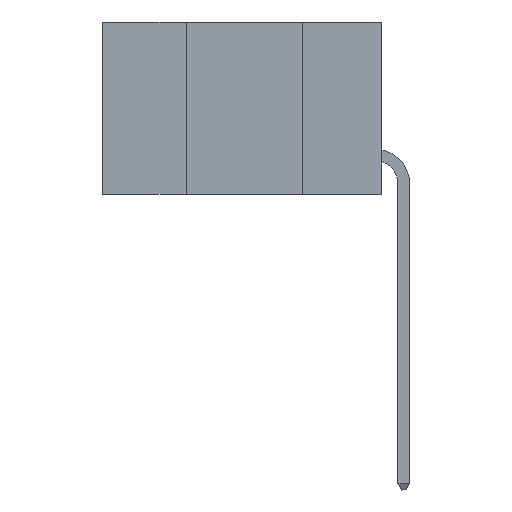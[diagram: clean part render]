
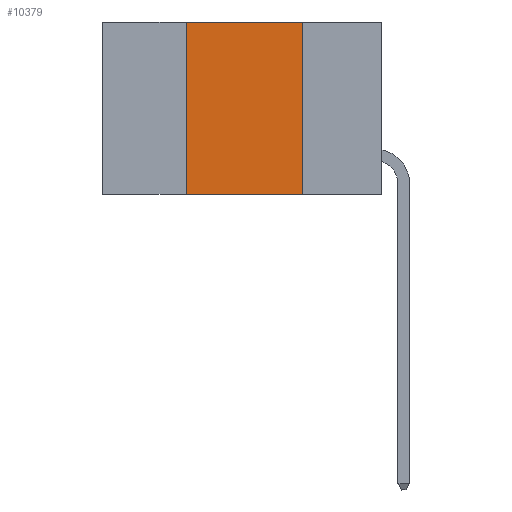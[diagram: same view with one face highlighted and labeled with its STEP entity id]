
A CAD part, left-side view. The second image highlights one B-rep face of the part: STEP entity #10379.
In plain terms, the highlighted planar face has unit normal (-1, 0, 0).
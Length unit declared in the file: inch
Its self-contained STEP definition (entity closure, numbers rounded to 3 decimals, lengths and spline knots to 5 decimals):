
#261 = DIRECTION ( 'NONE',  ( 0., 0., -1. ) ) ;
#329 = VECTOR ( 'NONE', #6479, 39.37008 ) ;
#475 = EDGE_CURVE ( 'NONE', #13426, #1788, #13228, .T. ) ;
#1064 = CARTESIAN_POINT ( 'NONE',  ( 0., 0.17, -0.37 ) ) ;
#1123 = EDGE_CURVE ( 'NONE', #13426, #13877, #6377, .T. ) ;
#1788 = VERTEX_POINT ( 'NONE', #1064 ) ;
#2422 = DIRECTION ( 'NONE',  ( 0., -1., 0. ) ) ;
#2506 = VERTEX_POINT ( 'NONE', #7104 ) ;
#3003 = CARTESIAN_POINT ( 'NONE',  ( 0., 0.42, -0.37 ) ) ;
#3726 = VECTOR ( 'NONE', #2422, 39.37008 ) ;
#3855 = PLANE ( 'NONE',  #8556 ) ;
#3953 = CARTESIAN_POINT ( 'NONE',  ( 0., 0.6, 0. ) ) ;
#4496 = ORIENTED_EDGE ( 'NONE', *, *, #13696, .F. ) ;
#4792 = DIRECTION ( 'NONE',  ( 0., 0., -1. ) ) ;
#4890 = DIRECTION ( 'NONE',  ( 1., 0., 0. ) ) ;
#6045 = ORIENTED_EDGE ( 'NONE', *, *, #1123, .F. ) ;
#6097 = VECTOR ( 'NONE', #261, 39.37008 ) ;
#6141 = CARTESIAN_POINT ( 'NONE',  ( 0., 0.6, -0.37 ) ) ;
#6282 = ORIENTED_EDGE ( 'NONE', *, *, #11385, .F. ) ;
#6344 = VECTOR ( 'NONE', #12982, 39.37008 ) ;
#6377 = LINE ( 'NONE', #7523, #329 ) ;
#6479 = DIRECTION ( 'NONE',  ( 0., 0., 1. ) ) ;
#7104 = CARTESIAN_POINT ( 'NONE',  ( 0., 0.17, 0. ) ) ;
#7523 = CARTESIAN_POINT ( 'NONE',  ( 0., 0.42, 0. ) ) ;
#7703 = CARTESIAN_POINT ( 'NONE',  ( 0., 0.6, 0. ) ) ;
#8556 = AXIS2_PLACEMENT_3D ( 'NONE', #3953, #4890, #4792 ) ;
#8904 = LINE ( 'NONE', #10072, #6097 ) ;
#9580 = EDGE_LOOP ( 'NONE', ( #6282, #4496, #6045, #9629 ) ) ;
#9629 = ORIENTED_EDGE ( 'NONE', *, *, #475, .T. ) ;
#10072 = CARTESIAN_POINT ( 'NONE',  ( 0., 0.17, 0. ) ) ;
#10379 = ADVANCED_FACE ( 'NONE', ( #11628 ), #3855, .F. ) ;
#11262 = CARTESIAN_POINT ( 'NONE',  ( 0., 0.42, 0. ) ) ;
#11385 = EDGE_CURVE ( 'NONE', #2506, #1788, #8904, .T. ) ;
#11628 = FACE_OUTER_BOUND ( 'NONE', #9580, .T. ) ;
#12982 = DIRECTION ( 'NONE',  ( 0., -1., 0. ) ) ;
#13228 = LINE ( 'NONE', #6141, #3726 ) ;
#13426 = VERTEX_POINT ( 'NONE', #3003 ) ;
#13672 = LINE ( 'NONE', #7703, #6344 ) ;
#13696 = EDGE_CURVE ( 'NONE', #13877, #2506, #13672, .T. ) ;
#13877 = VERTEX_POINT ( 'NONE', #11262 ) ;
